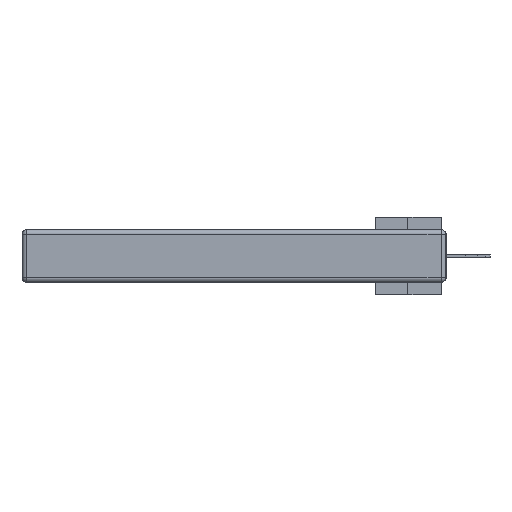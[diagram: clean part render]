
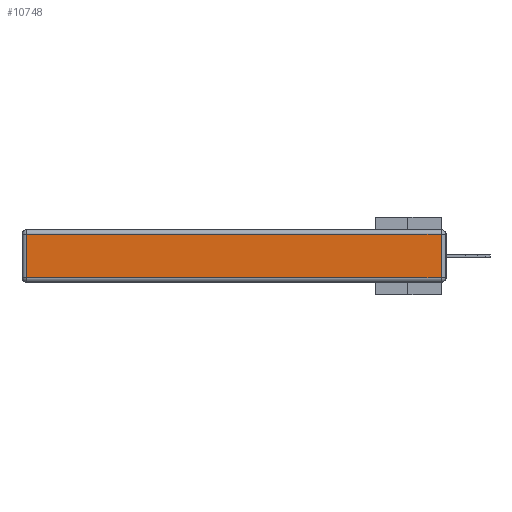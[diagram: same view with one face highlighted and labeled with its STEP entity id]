
A CAD part, left-side view. The second image highlights one B-rep face of the part: STEP entity #10748.
In plain terms, the highlighted planar face has unit normal (-1, 0, 0).
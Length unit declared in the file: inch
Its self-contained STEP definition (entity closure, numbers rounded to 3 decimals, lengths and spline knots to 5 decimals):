
#302 = VERTEX_POINT ( 'NONE', #8435 ) ;
#569 = VERTEX_POINT ( 'NONE', #30727 ) ;
#3952 = CARTESIAN_POINT ( 'NONE',  ( 0., 2.75, -0.03 ) ) ;
#4480 = PLANE ( 'NONE',  #21613 ) ;
#4668 = EDGE_CURVE ( 'NONE', #27100, #302, #6800, .T. ) ;
#5176 = VERTEX_POINT ( 'NONE', #28143 ) ;
#5861 = ORIENTED_EDGE ( 'NONE', *, *, #16743, .T. ) ;
#6215 = VECTOR ( 'NONE', #22640, 39.37008 ) ;
#6800 = LINE ( 'NONE', #16547, #10702 ) ;
#7348 = CARTESIAN_POINT ( 'NONE',  ( 0., 2.72, -0.313 ) ) ;
#8435 = CARTESIAN_POINT ( 'NONE',  ( 0., 0.03, -0.313 ) ) ;
#9393 = DIRECTION ( 'NONE',  ( -1., 0., 0. ) ) ;
#9708 = LINE ( 'NONE', #12142, #16036 ) ;
#10268 = VECTOR ( 'NONE', #23074, 39.37008 ) ;
#10702 = VECTOR ( 'NONE', #30641, 39.37008 ) ;
#10748 = ADVANCED_FACE ( 'NONE', ( #26207 ), #4480, .T. ) ;
#11685 = EDGE_CURVE ( 'NONE', #5176, #27100, #12644, .T. ) ;
#11930 = ORIENTED_EDGE ( 'NONE', *, *, #4668, .T. ) ;
#12142 = CARTESIAN_POINT ( 'NONE',  ( 0., 0.03, -0.343 ) ) ;
#12644 = LINE ( 'NONE', #15514, #6215 ) ;
#15514 = CARTESIAN_POINT ( 'NONE',  ( 0., 2.72, -0.343 ) ) ;
#16036 = VECTOR ( 'NONE', #26239, 39.37008 ) ;
#16118 = ORIENTED_EDGE ( 'NONE', *, *, #11685, .T. ) ;
#16199 = EDGE_LOOP ( 'NONE', ( #11930, #5861, #25903, #16118 ) ) ;
#16547 = CARTESIAN_POINT ( 'NONE',  ( 0., 0., -0.313 ) ) ;
#16743 = EDGE_CURVE ( 'NONE', #302, #569, #9708, .T. ) ;
#18989 = EDGE_CURVE ( 'NONE', #569, #5176, #28329, .T. ) ;
#21613 = AXIS2_PLACEMENT_3D ( 'NONE', #23592, #9393, #25922 ) ;
#22640 = DIRECTION ( 'NONE',  ( 0., 0., -1. ) ) ;
#23074 = DIRECTION ( 'NONE',  ( 0., 1., 0. ) ) ;
#23592 = CARTESIAN_POINT ( 'NONE',  ( 0., 0., -0.343 ) ) ;
#25903 = ORIENTED_EDGE ( 'NONE', *, *, #18989, .T. ) ;
#25922 = DIRECTION ( 'NONE',  ( 0., 0., 1. ) ) ;
#26207 = FACE_OUTER_BOUND ( 'NONE', #16199, .T. ) ;
#26239 = DIRECTION ( 'NONE',  ( 0., 0., 1. ) ) ;
#27100 = VERTEX_POINT ( 'NONE', #7348 ) ;
#28143 = CARTESIAN_POINT ( 'NONE',  ( 0., 2.72, -0.03 ) ) ;
#28329 = LINE ( 'NONE', #3952, #10268 ) ;
#30641 = DIRECTION ( 'NONE',  ( 0., -1., 0. ) ) ;
#30727 = CARTESIAN_POINT ( 'NONE',  ( 0., 0.03, -0.03 ) ) ;
